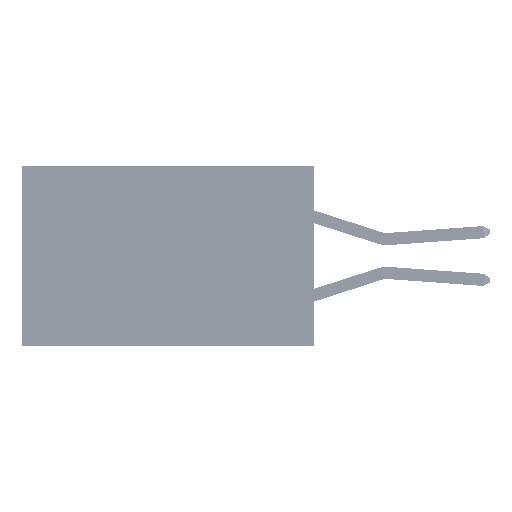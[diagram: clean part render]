
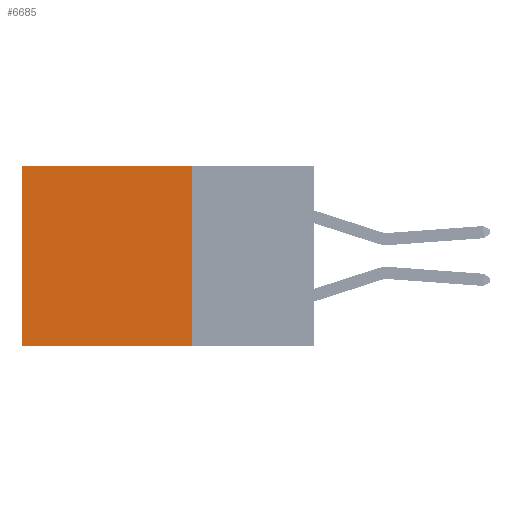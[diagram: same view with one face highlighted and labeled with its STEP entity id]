
A CAD part, left-side view. The second image highlights one B-rep face of the part: STEP entity #6685.
In plain terms, the highlighted planar face has unit normal (-1, 0, 0).
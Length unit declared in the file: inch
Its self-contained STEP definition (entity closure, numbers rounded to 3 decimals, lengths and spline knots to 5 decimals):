
#331 = CARTESIAN_POINT ( 'NONE',  ( 0.2875, 0.25, -0.37 ) ) ;
#1035 = VECTOR ( 'NONE', #25738, 39.37008 ) ;
#1885 = ORIENTED_EDGE ( 'NONE', *, *, #45502, .F. ) ;
#3508 = CARTESIAN_POINT ( 'NONE',  ( 0.2875, 0.25, -0.37 ) ) ;
#3694 = DIRECTION ( 'NONE',  ( 0., 0., -1. ) ) ;
#5289 = VERTEX_POINT ( 'NONE', #22342 ) ;
#6449 = VECTOR ( 'NONE', #7295, 39.37008 ) ;
#6685 = ADVANCED_FACE ( 'NONE', ( #14364 ), #44336, .F. ) ;
#7295 = DIRECTION ( 'NONE',  ( 0., 1., 0. ) ) ;
#7359 = LINE ( 'NONE', #35225, #45512 ) ;
#10972 = CARTESIAN_POINT ( 'NONE',  ( 0.2875, 0.25, 0. ) ) ;
#11615 = AXIS2_PLACEMENT_3D ( 'NONE', #22388, #26147, #3694 ) ;
#14364 = FACE_OUTER_BOUND ( 'NONE', #25181, .T. ) ;
#15102 = EDGE_CURVE ( 'NONE', #30988, #24660, #36198, .T. ) ;
#17358 = ORIENTED_EDGE ( 'NONE', *, *, #18858, .T. ) ;
#17976 = VERTEX_POINT ( 'NONE', #42915 ) ;
#18858 = EDGE_CURVE ( 'NONE', #5289, #24660, #22146, .T. ) ;
#20469 = DIRECTION ( 'NONE',  ( 0., 1., 0. ) ) ;
#20939 = EDGE_CURVE ( 'NONE', #17976, #5289, #7359, .T. ) ;
#21021 = ORIENTED_EDGE ( 'NONE', *, *, #20939, .T. ) ;
#22146 = LINE ( 'NONE', #40199, #1035 ) ;
#22155 = VECTOR ( 'NONE', #40475, 39.37008 ) ;
#22342 = CARTESIAN_POINT ( 'NONE',  ( 0.2875, 0.6, 0. ) ) ;
#22388 = CARTESIAN_POINT ( 'NONE',  ( 0.2875, 0.25, 0. ) ) ;
#24660 = VERTEX_POINT ( 'NONE', #37462 ) ;
#25181 = EDGE_LOOP ( 'NONE', ( #17358, #32986, #1885, #21021 ) ) ;
#25738 = DIRECTION ( 'NONE',  ( 0., 0., -1. ) ) ;
#26147 = DIRECTION ( 'NONE',  ( 1., 0., 0. ) ) ;
#30988 = VERTEX_POINT ( 'NONE', #331 ) ;
#32008 = LINE ( 'NONE', #10972, #22155 ) ;
#32986 = ORIENTED_EDGE ( 'NONE', *, *, #15102, .F. ) ;
#35225 = CARTESIAN_POINT ( 'NONE',  ( 0.2875, 0.25, 0. ) ) ;
#36198 = LINE ( 'NONE', #3508, #6449 ) ;
#37462 = CARTESIAN_POINT ( 'NONE',  ( 0.2875, 0.6, -0.37 ) ) ;
#40199 = CARTESIAN_POINT ( 'NONE',  ( 0.2875, 0.6, 0. ) ) ;
#40475 = DIRECTION ( 'NONE',  ( 0., 0., -1. ) ) ;
#42915 = CARTESIAN_POINT ( 'NONE',  ( 0.2875, 0.25, 0. ) ) ;
#44336 = PLANE ( 'NONE',  #11615 ) ;
#45502 = EDGE_CURVE ( 'NONE', #17976, #30988, #32008, .T. ) ;
#45512 = VECTOR ( 'NONE', #20469, 39.37008 ) ;
